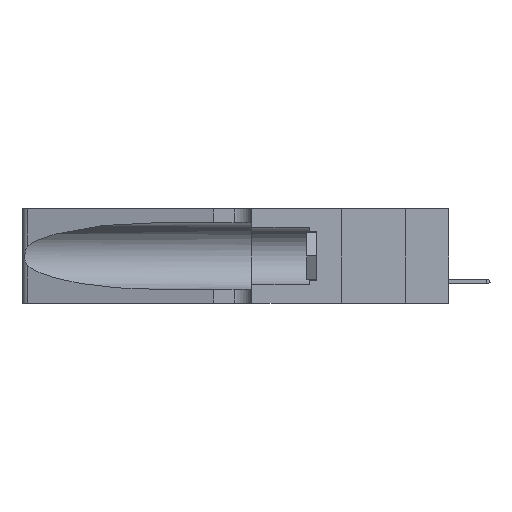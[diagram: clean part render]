
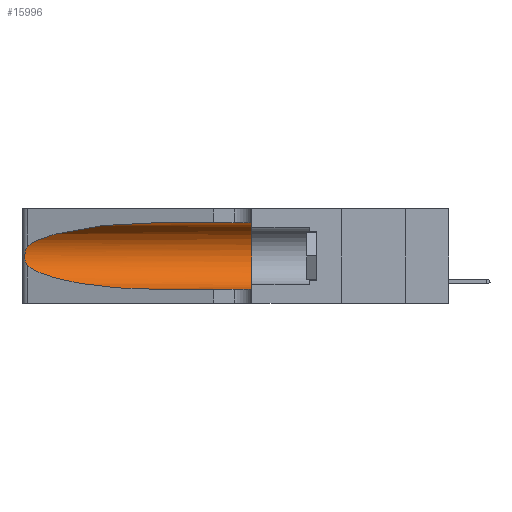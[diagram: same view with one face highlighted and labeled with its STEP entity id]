
A CAD part, left-side view. The second image highlights one B-rep face of the part: STEP entity #15996.
In plain terms, the highlighted cylindrical face has radius 3.308 mm (diameter 6.617 mm), a partial arc.
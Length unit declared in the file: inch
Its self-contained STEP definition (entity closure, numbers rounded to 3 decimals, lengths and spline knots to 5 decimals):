
#78 = DIRECTION ( 'NONE',  ( 0., 0., 1. ) ) ;
#629 =( BOUNDED_CURVE ( )  B_SPLINE_CURVE ( 3, ( #9925, #33040, #26451, #1717 ),
 .UNSPECIFIED., .F., .F. ) 
 B_SPLINE_CURVE_WITH_KNOTS ( ( 4, 4 ),
 ( 1.5708, 2.84003 ),
 .UNSPECIFIED. ) 
 CURVE ( )  GEOMETRIC_REPRESENTATION_ITEM ( )  RATIONAL_B_SPLINE_CURVE ( ( 1., 0.87, 0.87, 1. ) ) 
 REPRESENTATION_ITEM ( '' )  );
#1717 = CARTESIAN_POINT ( 'NONE',  ( 0.25487, 1.22718, 0.22369 ) ) ;
#2270 = VERTEX_POINT ( 'NONE', #20878 ) ;
#3350 = ORIENTED_EDGE ( 'NONE', *, *, #31565, .T. ) ;
#3929 = CARTESIAN_POINT ( 'NONE',  ( 0.26075, 1.23896, 0.19203 ) ) ;
#4053 = CARTESIAN_POINT ( 'NONE',  ( 0.25487, 1.22718, 0.14631 ) ) ;
#4518 = EDGE_CURVE ( 'NONE', #4885, #12088, #6463, .T. ) ;
#4885 = VERTEX_POINT ( 'NONE', #20269 ) ;
#5003 = CARTESIAN_POINT ( 'NONE',  ( 0.1305, 1.61858, 0.31525 ) ) ;
#5079 = CIRCLE ( 'NONE', #12491, 0.13025 ) ;
#6463 = LINE ( 'NONE', #5003, #11917 ) ;
#7333 = CARTESIAN_POINT ( 'NONE',  ( 0.25856, 1.23593, 0.16098 ) ) ;
#7440 = EDGE_CURVE ( 'NONE', #12088, #31829, #5079, .T. ) ;
#8088 = DIRECTION ( 'NONE',  ( 0., -1., 0. ) ) ;
#9925 = CARTESIAN_POINT ( 'NONE',  ( 0.1305, 0.72297, 0.31525 ) ) ;
#10191 = CARTESIAN_POINT ( 'NONE',  ( 0.18966, 0.96281, 0.05475 ) ) ;
#10611 = CYLINDRICAL_SURFACE ( 'NONE', #36942, 0.13025 ) ;
#11644 = FACE_OUTER_BOUND ( 'NONE', #34522, .T. ) ;
#11760 = VECTOR ( 'NONE', #24950, 39.37008 ) ;
#11917 = VECTOR ( 'NONE', #33317, 39.37008 ) ;
#12088 = VERTEX_POINT ( 'NONE', #14264 ) ;
#12491 = AXIS2_PLACEMENT_3D ( 'NONE', #28249, #31161, #78 ) ;
#13678 = CARTESIAN_POINT ( 'NONE',  ( 0.26075, 1.23896, 0.178 ) ) ;
#14264 = CARTESIAN_POINT ( 'NONE',  ( 0.1305, 0.35, 0.31525 ) ) ;
#15273 = B_SPLINE_CURVE_WITH_KNOTS ( 'NONE', 3,
 ( #32509, #23312, #29620, #17127, #26199, #22759, #3929, #13678, #32367, #7333, #38577, #25928, #19740, #4053 ),
 .UNSPECIFIED., .F., .F.,
 ( 4, 2, 2, 2, 2, 2, 4 ),
 ( 0., 0.00027, 0.00053, 0.00107, 0.0016, 0.00187, 0.00214 ),
 .UNSPECIFIED. ) ;
#15996 = ADVANCED_FACE ( 'NONE', ( #11644 ), #10611, .F. ) ;
#17127 = CARTESIAN_POINT ( 'NONE',  ( 0.25787, 1.23484, 0.2124 ) ) ;
#17468 = CARTESIAN_POINT ( 'NONE',  ( 0.1305, 0.35, 0.05475 ) ) ;
#18447 = ORIENTED_EDGE ( 'NONE', *, *, #7440, .F. ) ;
#19549 =( BOUNDED_CURVE ( )  B_SPLINE_CURVE ( 3, ( #29046, #26178, #10191, #35376 ),
 .UNSPECIFIED., .F., .F. ) 
 B_SPLINE_CURVE_WITH_KNOTS ( ( 4, 4 ),
 ( 3.44316, 4.71239 ),
 .UNSPECIFIED. ) 
 CURVE ( )  GEOMETRIC_REPRESENTATION_ITEM ( )  RATIONAL_B_SPLINE_CURVE ( ( 1., 0.87, 0.87, 1. ) ) 
 REPRESENTATION_ITEM ( '' )  );
#19553 = CARTESIAN_POINT ( 'NONE',  ( 0.25487, 1.22718, 0.14631 ) ) ;
#19740 = CARTESIAN_POINT ( 'NONE',  ( 0.25555, 1.22993, 0.14849 ) ) ;
#20269 = CARTESIAN_POINT ( 'NONE',  ( 0.1305, 0.72297, 0.31525 ) ) ;
#20878 = CARTESIAN_POINT ( 'NONE',  ( 0.25487, 1.22718, 0.22369 ) ) ;
#21821 = VERTEX_POINT ( 'NONE', #19553 ) ;
#22759 = CARTESIAN_POINT ( 'NONE',  ( 0.26018, 1.23835, 0.19895 ) ) ;
#22842 = EDGE_CURVE ( 'NONE', #4885, #2270, #629, .T. ) ;
#23312 = CARTESIAN_POINT ( 'NONE',  ( 0.25555, 1.22994, 0.2215 ) ) ;
#23804 = CARTESIAN_POINT ( 'NONE',  ( 0.1305, 1.61858, 0.185 ) ) ;
#24950 = DIRECTION ( 'NONE',  ( 0., -1., 0. ) ) ;
#25928 = CARTESIAN_POINT ( 'NONE',  ( 0.25639, 1.23186, 0.15144 ) ) ;
#26178 = CARTESIAN_POINT ( 'NONE',  ( 0.2373, 1.15595, 0.08982 ) ) ;
#26199 = CARTESIAN_POINT ( 'NONE',  ( 0.25854, 1.2359, 0.20912 ) ) ;
#26451 = CARTESIAN_POINT ( 'NONE',  ( 0.2373, 1.15595, 0.28018 ) ) ;
#26907 = VERTEX_POINT ( 'NONE', #27814 ) ;
#27814 = CARTESIAN_POINT ( 'NONE',  ( 0.1305, 0.72297, 0.05475 ) ) ;
#28249 = CARTESIAN_POINT ( 'NONE',  ( 0.1305, 0.35, 0.185 ) ) ;
#28438 = LINE ( 'NONE', #40100, #11760 ) ;
#29046 = CARTESIAN_POINT ( 'NONE',  ( 0.25487, 1.22718, 0.14631 ) ) ;
#29620 = CARTESIAN_POINT ( 'NONE',  ( 0.25639, 1.23184, 0.21858 ) ) ;
#30103 = DIRECTION ( 'NONE',  ( 0., 0., -1. ) ) ;
#30523 = EDGE_CURVE ( 'NONE', #21821, #26907, #19549, .T. ) ;
#31161 = DIRECTION ( 'NONE',  ( 0., 1., 0. ) ) ;
#31565 = EDGE_CURVE ( 'NONE', #26907, #31829, #28438, .T. ) ;
#31829 = VERTEX_POINT ( 'NONE', #17468 ) ;
#32367 = CARTESIAN_POINT ( 'NONE',  ( 0.26017, 1.23833, 0.17102 ) ) ;
#32509 = CARTESIAN_POINT ( 'NONE',  ( 0.25487, 1.22718, 0.22369 ) ) ;
#33040 = CARTESIAN_POINT ( 'NONE',  ( 0.18966, 0.96281, 0.31525 ) ) ;
#33317 = DIRECTION ( 'NONE',  ( 0., -1., 0. ) ) ;
#34522 = EDGE_LOOP ( 'NONE', ( #37343, #39812, #39659, #3350, #18447, #40667 ) ) ;
#35376 = CARTESIAN_POINT ( 'NONE',  ( 0.1305, 0.72297, 0.05475 ) ) ;
#36897 = EDGE_CURVE ( 'NONE', #2270, #21821, #15273, .T. ) ;
#36942 = AXIS2_PLACEMENT_3D ( 'NONE', #23804, #8088, #30103 ) ;
#37343 = ORIENTED_EDGE ( 'NONE', *, *, #22842, .T. ) ;
#38577 = CARTESIAN_POINT ( 'NONE',  ( 0.25789, 1.23486, 0.15765 ) ) ;
#39659 = ORIENTED_EDGE ( 'NONE', *, *, #30523, .T. ) ;
#39812 = ORIENTED_EDGE ( 'NONE', *, *, #36897, .T. ) ;
#40100 = CARTESIAN_POINT ( 'NONE',  ( 0.1305, 1.61858, 0.05475 ) ) ;
#40667 = ORIENTED_EDGE ( 'NONE', *, *, #4518, .F. ) ;
